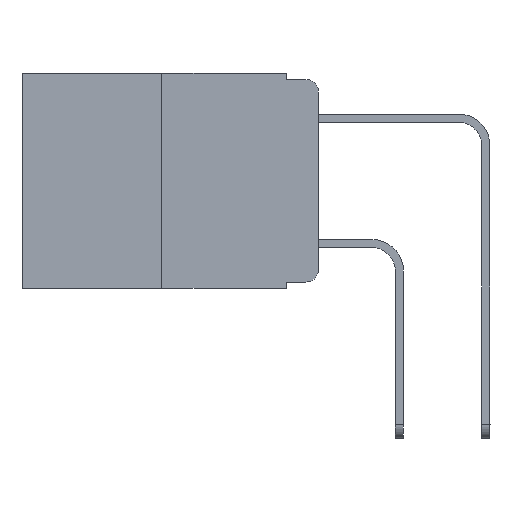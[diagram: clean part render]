
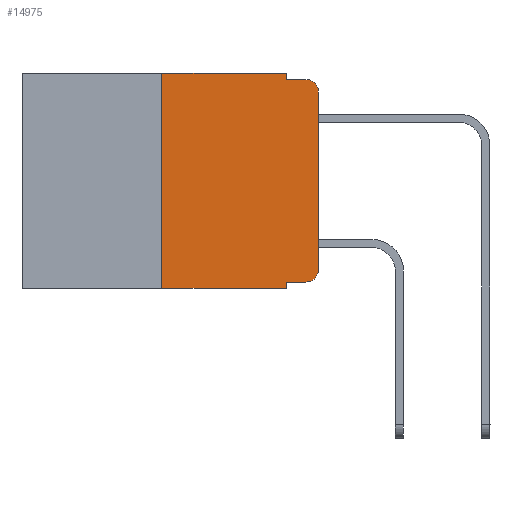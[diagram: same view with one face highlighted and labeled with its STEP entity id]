
A CAD part, left-side view. The second image highlights one B-rep face of the part: STEP entity #14975.
In plain terms, the highlighted planar face has unit normal (-1, 0, 0).
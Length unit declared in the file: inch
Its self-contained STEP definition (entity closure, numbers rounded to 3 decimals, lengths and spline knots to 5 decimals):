
#345 = CARTESIAN_POINT ( 'NONE',  ( 0., 0.051, -0.333 ) ) ;
#447 = DIRECTION ( 'NONE',  ( 0., 0., -1. ) ) ;
#509 = VERTEX_POINT ( 'NONE', #5056 ) ;
#665 = ORIENTED_EDGE ( 'NONE', *, *, #11168, .F. ) ;
#843 = AXIS2_PLACEMENT_3D ( 'NONE', #22261, #1061, #6480 ) ;
#1061 = DIRECTION ( 'NONE',  ( -1., 0., 0. ) ) ;
#1112 = CARTESIAN_POINT ( 'NONE',  ( 0., 0.25, 0. ) ) ;
#1741 = VERTEX_POINT ( 'NONE', #22278 ) ;
#1856 = DIRECTION ( 'NONE',  ( 0., -1., 0. ) ) ;
#2264 = FACE_OUTER_BOUND ( 'NONE', #21643, .T. ) ;
#2586 = CARTESIAN_POINT ( 'NONE',  ( 0., 0., -0.313 ) ) ;
#3143 = VECTOR ( 'NONE', #18406, 39.37008 ) ;
#3516 = CARTESIAN_POINT ( 'NONE',  ( 0., 0.051, -0.333 ) ) ;
#3589 = EDGE_CURVE ( 'NONE', #1741, #20931, #7946, .T. ) ;
#4929 = DIRECTION ( 'NONE',  ( -1., 0., 0. ) ) ;
#5017 = CARTESIAN_POINT ( 'NONE',  ( 0., 0.02, -0.333 ) ) ;
#5056 = CARTESIAN_POINT ( 'NONE',  ( 0., 0., -0.03 ) ) ;
#5109 = ORIENTED_EDGE ( 'NONE', *, *, #13985, .T. ) ;
#5406 = LINE ( 'NONE', #20185, #19907 ) ;
#5444 = DIRECTION ( 'NONE',  ( 0., -1., 0. ) ) ;
#6172 = LINE ( 'NONE', #1112, #12197 ) ;
#6480 = DIRECTION ( 'NONE',  ( 0., 0., -1. ) ) ;
#7038 = CARTESIAN_POINT ( 'NONE',  ( 0., 0.051, 0. ) ) ;
#7451 = CARTESIAN_POINT ( 'NONE',  ( 0., 0., 0. ) ) ;
#7555 = VERTEX_POINT ( 'NONE', #15295 ) ;
#7946 = LINE ( 'NONE', #15364, #14133 ) ;
#8216 = DIRECTION ( 'NONE',  ( 0., 0., 1. ) ) ;
#8375 = VERTEX_POINT ( 'NONE', #345 ) ;
#8548 = VECTOR ( 'NONE', #16678, 39.37008 ) ;
#8957 = CARTESIAN_POINT ( 'NONE',  ( 0., 0.051, -0.01 ) ) ;
#9494 = ORIENTED_EDGE ( 'NONE', *, *, #20173, .F. ) ;
#9615 = CARTESIAN_POINT ( 'NONE',  ( 0., 0.473, 0. ) ) ;
#9802 = VERTEX_POINT ( 'NONE', #15469 ) ;
#9842 = CARTESIAN_POINT ( 'NONE',  ( 0., 0.02, -0.01 ) ) ;
#10781 = LINE ( 'NONE', #8957, #13389 ) ;
#10880 = CIRCLE ( 'NONE', #843, 0.02 ) ;
#11031 = LINE ( 'NONE', #7038, #3143 ) ;
#11039 = DIRECTION ( 'NONE',  ( 0., 0., -1. ) ) ;
#11158 = CARTESIAN_POINT ( 'NONE',  ( 0., 0.473, 0. ) ) ;
#11168 = EDGE_CURVE ( 'NONE', #8375, #9802, #11031, .T. ) ;
#11547 = PLANE ( 'NONE',  #22145 ) ;
#11858 = EDGE_CURVE ( 'NONE', #19735, #16905, #10880, .T. ) ;
#12197 = VECTOR ( 'NONE', #8216, 39.37008 ) ;
#12402 = ORIENTED_EDGE ( 'NONE', *, *, #11858, .T. ) ;
#13389 = VECTOR ( 'NONE', #16369, 39.37008 ) ;
#13622 = EDGE_CURVE ( 'NONE', #16905, #509, #18472, .T. ) ;
#13985 = EDGE_CURVE ( 'NONE', #509, #22311, #18239, .T. ) ;
#14017 = EDGE_CURVE ( 'NONE', #22093, #1741, #18414, .T. ) ;
#14133 = VECTOR ( 'NONE', #22736, 39.37008 ) ;
#14165 = ORIENTED_EDGE ( 'NONE', *, *, #20242, .T. ) ;
#14251 = CARTESIAN_POINT ( 'NONE',  ( 0., 0.02, -0.03 ) ) ;
#14517 = DIRECTION ( 'NONE',  ( 0., -1., 0. ) ) ;
#14975 = ADVANCED_FACE ( 'NONE', ( #2264 ), #11547, .F. ) ;
#15168 = VECTOR ( 'NONE', #1856, 39.37008 ) ;
#15295 = CARTESIAN_POINT ( 'NONE',  ( 0., 0.25, -0.343 ) ) ;
#15364 = CARTESIAN_POINT ( 'NONE',  ( 0., 0.051, 0. ) ) ;
#15469 = CARTESIAN_POINT ( 'NONE',  ( 0., 0.051, -0.343 ) ) ;
#15498 = ORIENTED_EDGE ( 'NONE', *, *, #13622, .T. ) ;
#15568 = AXIS2_PLACEMENT_3D ( 'NONE', #14251, #4929, #11039 ) ;
#16369 = DIRECTION ( 'NONE',  ( 0., -1., 0. ) ) ;
#16678 = DIRECTION ( 'NONE',  ( 0., 0., 1. ) ) ;
#16872 = VECTOR ( 'NONE', #5444, 39.37008 ) ;
#16905 = VERTEX_POINT ( 'NONE', #2586 ) ;
#17009 = DIRECTION ( 'NONE',  ( 1., 0., 0. ) ) ;
#17136 = ORIENTED_EDGE ( 'NONE', *, *, #18973, .T. ) ;
#17469 = EDGE_CURVE ( 'NONE', #7555, #22093, #6172, .T. ) ;
#18239 = CIRCLE ( 'NONE', #15568, 0.02 ) ;
#18406 = DIRECTION ( 'NONE',  ( 0., 0., -1. ) ) ;
#18414 = LINE ( 'NONE', #11158, #15168 ) ;
#18472 = LINE ( 'NONE', #7451, #8548 ) ;
#18514 = LINE ( 'NONE', #3516, #16872 ) ;
#18973 = EDGE_CURVE ( 'NONE', #7555, #9802, #5406, .T. ) ;
#19101 = CARTESIAN_POINT ( 'NONE',  ( 0., 0.25, 0. ) ) ;
#19735 = VERTEX_POINT ( 'NONE', #5017 ) ;
#19907 = VECTOR ( 'NONE', #14517, 39.37008 ) ;
#20173 = EDGE_CURVE ( 'NONE', #20931, #22311, #10781, .T. ) ;
#20185 = CARTESIAN_POINT ( 'NONE',  ( 0., 0.473, -0.343 ) ) ;
#20242 = EDGE_CURVE ( 'NONE', #8375, #19735, #18514, .T. ) ;
#20422 = ORIENTED_EDGE ( 'NONE', *, *, #17469, .F. ) ;
#20806 = ORIENTED_EDGE ( 'NONE', *, *, #3589, .F. ) ;
#20931 = VERTEX_POINT ( 'NONE', #23893 ) ;
#21643 = EDGE_LOOP ( 'NONE', ( #15498, #5109, #9494, #20806, #22313, #20422, #17136, #665, #14165, #12402 ) ) ;
#22093 = VERTEX_POINT ( 'NONE', #19101 ) ;
#22145 = AXIS2_PLACEMENT_3D ( 'NONE', #9615, #17009, #447 ) ;
#22261 = CARTESIAN_POINT ( 'NONE',  ( 0., 0.02, -0.313 ) ) ;
#22278 = CARTESIAN_POINT ( 'NONE',  ( 0., 0.051, 0. ) ) ;
#22311 = VERTEX_POINT ( 'NONE', #9842 ) ;
#22313 = ORIENTED_EDGE ( 'NONE', *, *, #14017, .F. ) ;
#22736 = DIRECTION ( 'NONE',  ( 0., 0., -1. ) ) ;
#23893 = CARTESIAN_POINT ( 'NONE',  ( 0., 0.051, -0.01 ) ) ;
